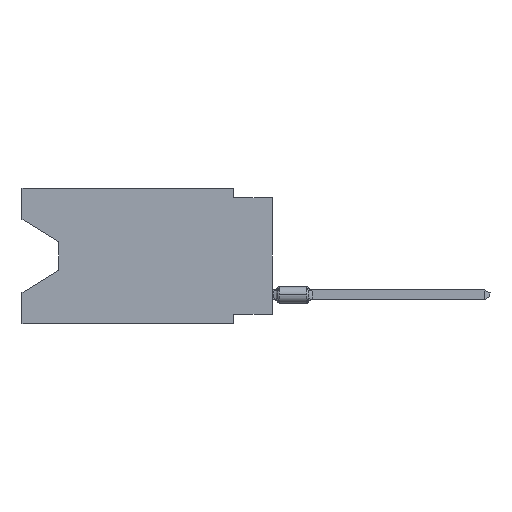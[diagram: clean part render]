
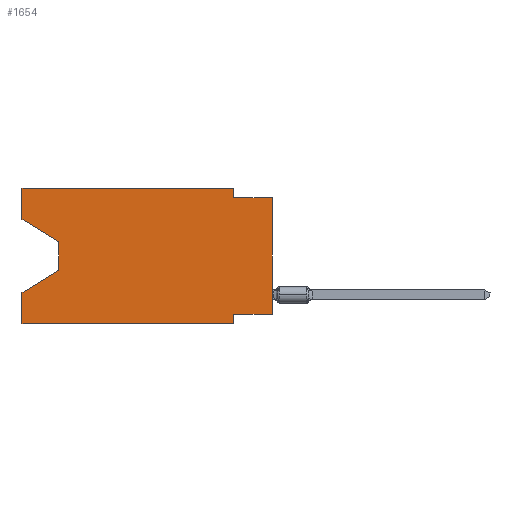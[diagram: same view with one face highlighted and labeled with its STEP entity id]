
A CAD part, left-side view. The second image highlights one B-rep face of the part: STEP entity #1654.
In plain terms, the highlighted planar face has unit normal (-1, 0, 0).
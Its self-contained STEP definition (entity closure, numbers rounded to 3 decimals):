
#475 = VECTOR ( 'NONE', #41238, 1000. ) ;
#774 = VERTEX_POINT ( 'NONE', #34851 ) ;
#920 = VECTOR ( 'NONE', #32860, 1000. ) ;
#998 = CARTESIAN_POINT ( 'NONE',  ( 0., 16.383, 0. ) ) ;
#1012 = VERTEX_POINT ( 'NONE', #33059 ) ;
#1635 = DIRECTION ( 'NONE',  ( 0., 0., -1. ) ) ;
#1654 = ADVANCED_FACE ( 'NONE', ( #1842 ), #4523, .F. ) ;
#1724 = LINE ( 'NONE', #18707, #475 ) ;
#1842 = FACE_OUTER_BOUND ( 'NONE', #28139, .T. ) ;
#2073 = ORIENTED_EDGE ( 'NONE', *, *, #21433, .F. ) ;
#2564 = ORIENTED_EDGE ( 'NONE', *, *, #16298, .F. ) ;
#2702 = LINE ( 'NONE', #3125, #33391 ) ;
#2910 = CARTESIAN_POINT ( 'NONE',  ( 0., 16.383, -6.852 ) ) ;
#3125 = CARTESIAN_POINT ( 'NONE',  ( 0., 2.54, 0. ) ) ;
#4424 = EDGE_CURVE ( 'NONE', #25284, #10142, #1724, .T. ) ;
#4523 = PLANE ( 'NONE',  #35125 ) ;
#4886 = CARTESIAN_POINT ( 'NONE',  ( 0., 2.54, 0. ) ) ;
#5183 = VERTEX_POINT ( 'NONE', #2910 ) ;
#5586 = EDGE_CURVE ( 'NONE', #8378, #774, #37267, .T. ) ;
#5741 = LINE ( 'NONE', #36607, #12336 ) ;
#6369 = VECTOR ( 'NONE', #42109, 1000. ) ;
#7306 = EDGE_CURVE ( 'NONE', #25980, #5183, #27415, .T. ) ;
#8145 = CARTESIAN_POINT ( 'NONE',  ( 0., 16.383, -8.89 ) ) ;
#8378 = VERTEX_POINT ( 'NONE', #25463 ) ;
#10016 = LINE ( 'NONE', #13099, #18811 ) ;
#10142 = VERTEX_POINT ( 'NONE', #30392 ) ;
#10559 = VECTOR ( 'NONE', #17483, 1000. ) ;
#11258 = LINE ( 'NONE', #35052, #11858 ) ;
#11858 = VECTOR ( 'NONE', #38169, 1000. ) ;
#12336 = VECTOR ( 'NONE', #16309, 1000. ) ;
#12509 = LINE ( 'NONE', #22865, #42012 ) ;
#13099 = CARTESIAN_POINT ( 'NONE',  ( 0., 16.383, 0. ) ) ;
#13660 = EDGE_CURVE ( 'NONE', #10142, #5183, #21157, .T. ) ;
#13887 = CARTESIAN_POINT ( 'NONE',  ( 0., 0., 0. ) ) ;
#14188 = EDGE_CURVE ( 'NONE', #23796, #37113, #2702, .T. ) ;
#14876 = DIRECTION ( 'NONE',  ( 1., 0., 0. ) ) ;
#15403 = EDGE_CURVE ( 'NONE', #31781, #23796, #5741, .T. ) ;
#16298 = EDGE_CURVE ( 'NONE', #18017, #31781, #10016, .T. ) ;
#16309 = DIRECTION ( 'NONE',  ( 0., -1., 0. ) ) ;
#17179 = VECTOR ( 'NONE', #18493, 1000. ) ;
#17483 = DIRECTION ( 'NONE',  ( 0., 0., 1. ) ) ;
#17995 = CARTESIAN_POINT ( 'NONE',  ( 0., 2.54, -8.89 ) ) ;
#18017 = VERTEX_POINT ( 'NONE', #27604 ) ;
#18275 = CARTESIAN_POINT ( 'NONE',  ( 0., 13.97, -5.385 ) ) ;
#18309 = VECTOR ( 'NONE', #41264, 1000. ) ;
#18493 = DIRECTION ( 'NONE',  ( 0., 0.855, -0.519 ) ) ;
#18677 = DIRECTION ( 'NONE',  ( 0., 1., 0. ) ) ;
#18707 = CARTESIAN_POINT ( 'NONE',  ( 0., 13.97, -3.505 ) ) ;
#18811 = VECTOR ( 'NONE', #43325, 1000. ) ;
#19592 = CARTESIAN_POINT ( 'NONE',  ( 0., 16.383, 0. ) ) ;
#20123 = EDGE_CURVE ( 'NONE', #18017, #25284, #11258, .T. ) ;
#20134 = CARTESIAN_POINT ( 'NONE',  ( 0., 16.383, 0. ) ) ;
#21157 = LINE ( 'NONE', #18275, #17179 ) ;
#21433 = EDGE_CURVE ( 'NONE', #37113, #774, #30904, .T. ) ;
#21808 = CARTESIAN_POINT ( 'NONE',  ( 0., 16.383, -8.89 ) ) ;
#22865 = CARTESIAN_POINT ( 'NONE',  ( 0., 0., -8.255 ) ) ;
#23155 = DIRECTION ( 'NONE',  ( 0., 0., 1. ) ) ;
#23796 = VERTEX_POINT ( 'NONE', #4886 ) ;
#25036 = ORIENTED_EDGE ( 'NONE', *, *, #14188, .F. ) ;
#25284 = VERTEX_POINT ( 'NONE', #27314 ) ;
#25463 = CARTESIAN_POINT ( 'NONE',  ( 0., 0., -8.255 ) ) ;
#25953 = EDGE_CURVE ( 'NONE', #25980, #36075, #28640, .T. ) ;
#25980 = VERTEX_POINT ( 'NONE', #8145 ) ;
#26423 = ORIENTED_EDGE ( 'NONE', *, *, #43105, .F. ) ;
#27314 = CARTESIAN_POINT ( 'NONE',  ( 0., 13.97, -3.505 ) ) ;
#27415 = LINE ( 'NONE', #20134, #10559 ) ;
#27604 = CARTESIAN_POINT ( 'NONE',  ( 0., 16.383, -2.038 ) ) ;
#28071 = CARTESIAN_POINT ( 'NONE',  ( 0., 2.54, -0.635 ) ) ;
#28139 = EDGE_LOOP ( 'NONE', ( #38842, #42293, #31931, #43389, #32605, #26423, #38566, #28812, #2073, #25036, #35864, #2564 ) ) ;
#28640 = LINE ( 'NONE', #21808, #6369 ) ;
#28812 = ORIENTED_EDGE ( 'NONE', *, *, #5586, .T. ) ;
#30392 = CARTESIAN_POINT ( 'NONE',  ( 0., 13.97, -5.385 ) ) ;
#30904 = LINE ( 'NONE', #37738, #18309 ) ;
#31781 = VERTEX_POINT ( 'NONE', #19592 ) ;
#31931 = ORIENTED_EDGE ( 'NONE', *, *, #13660, .T. ) ;
#32605 = ORIENTED_EDGE ( 'NONE', *, *, #25953, .T. ) ;
#32860 = DIRECTION ( 'NONE',  ( 0., 0., -1. ) ) ;
#33059 = CARTESIAN_POINT ( 'NONE',  ( 0., 2.54, -8.255 ) ) ;
#33391 = VECTOR ( 'NONE', #36024, 1000. ) ;
#34851 = CARTESIAN_POINT ( 'NONE',  ( 0., 0., -0.635 ) ) ;
#35052 = CARTESIAN_POINT ( 'NONE',  ( 0., 16.383, -2.038 ) ) ;
#35125 = AXIS2_PLACEMENT_3D ( 'NONE', #998, #14876, #1635 ) ;
#35864 = ORIENTED_EDGE ( 'NONE', *, *, #15403, .F. ) ;
#36024 = DIRECTION ( 'NONE',  ( 0., 0., -1. ) ) ;
#36075 = VERTEX_POINT ( 'NONE', #17995 ) ;
#36169 = LINE ( 'NONE', #43011, #920 ) ;
#36607 = CARTESIAN_POINT ( 'NONE',  ( 0., 16.383, 0. ) ) ;
#37113 = VERTEX_POINT ( 'NONE', #28071 ) ;
#37267 = LINE ( 'NONE', #13887, #41442 ) ;
#37738 = CARTESIAN_POINT ( 'NONE',  ( 0., 0., -0.635 ) ) ;
#38169 = DIRECTION ( 'NONE',  ( 0., -0.855, -0.519 ) ) ;
#38566 = ORIENTED_EDGE ( 'NONE', *, *, #43442, .F. ) ;
#38842 = ORIENTED_EDGE ( 'NONE', *, *, #20123, .T. ) ;
#41238 = DIRECTION ( 'NONE',  ( 0., 0., -1. ) ) ;
#41264 = DIRECTION ( 'NONE',  ( 0., -1., 0. ) ) ;
#41442 = VECTOR ( 'NONE', #23155, 1000. ) ;
#42012 = VECTOR ( 'NONE', #18677, 1000. ) ;
#42109 = DIRECTION ( 'NONE',  ( 0., -1., 0. ) ) ;
#42293 = ORIENTED_EDGE ( 'NONE', *, *, #4424, .T. ) ;
#43011 = CARTESIAN_POINT ( 'NONE',  ( 0., 2.54, -8.89 ) ) ;
#43105 = EDGE_CURVE ( 'NONE', #1012, #36075, #36169, .T. ) ;
#43325 = DIRECTION ( 'NONE',  ( 0., 0., 1. ) ) ;
#43389 = ORIENTED_EDGE ( 'NONE', *, *, #7306, .F. ) ;
#43442 = EDGE_CURVE ( 'NONE', #8378, #1012, #12509, .T. ) ;
